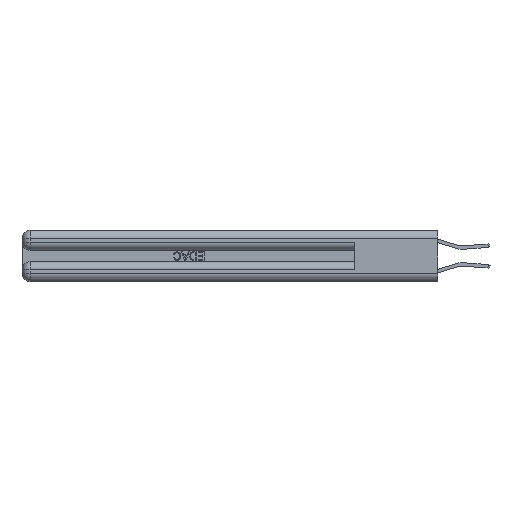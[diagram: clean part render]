
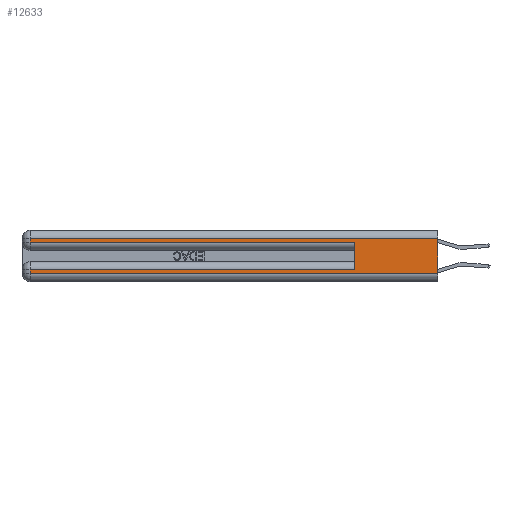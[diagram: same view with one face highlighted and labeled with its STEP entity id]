
A CAD part, left-side view. The second image highlights one B-rep face of the part: STEP entity #12633.
In plain terms, the highlighted planar face has unit normal (-1, 0, 0).
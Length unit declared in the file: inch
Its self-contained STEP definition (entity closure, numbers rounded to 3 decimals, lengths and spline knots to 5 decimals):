
#462 = FACE_OUTER_BOUND ( 'NONE', #24017, .T. ) ;
#1166 = LINE ( 'NONE', #32086, #22992 ) ;
#1452 = DIRECTION ( 'NONE',  ( 0., 1., 0. ) ) ;
#1502 = DIRECTION ( 'NONE',  ( 1., 0., 0. ) ) ;
#1860 = VERTEX_POINT ( 'NONE', #12380 ) ;
#1952 = EDGE_CURVE ( 'NONE', #29639, #1860, #1166, .T. ) ;
#2369 = VERTEX_POINT ( 'NONE', #33771 ) ;
#2550 = DIRECTION ( 'NONE',  ( 0., 0., 1. ) ) ;
#3182 = EDGE_CURVE ( 'NONE', #1860, #25771, #23637, .T. ) ;
#3885 = VECTOR ( 'NONE', #21975, 39.37008 ) ;
#4434 = DIRECTION ( 'NONE',  ( 0., 0., -1. ) ) ;
#5107 = LINE ( 'NONE', #13346, #8447 ) ;
#5162 = VECTOR ( 'NONE', #10854, 39.37008 ) ;
#5503 = ORIENTED_EDGE ( 'NONE', *, *, #1952, .T. ) ;
#5693 = LINE ( 'NONE', #18627, #14894 ) ;
#6251 = ORIENTED_EDGE ( 'NONE', *, *, #6834, .T. ) ;
#6834 = EDGE_CURVE ( 'NONE', #17349, #29639, #7426, .T. ) ;
#6919 = CARTESIAN_POINT ( 'NONE',  ( 0., 0., 0.37 ) ) ;
#7426 = LINE ( 'NONE', #16946, #18758 ) ;
#8447 = VECTOR ( 'NONE', #13696, 39.37008 ) ;
#8939 = VECTOR ( 'NONE', #26498, 39.37008 ) ;
#9323 = CARTESIAN_POINT ( 'NONE',  ( 0., 2.94, 0.285 ) ) ;
#9407 = LINE ( 'NONE', #28762, #27426 ) ;
#10305 = EDGE_CURVE ( 'NONE', #17349, #32527, #5693, .T. ) ;
#10809 = EDGE_CURVE ( 'NONE', #22746, #25771, #9407, .T. ) ;
#10854 = DIRECTION ( 'NONE',  ( 0., -1., 0. ) ) ;
#11839 = LINE ( 'NONE', #31795, #8939 ) ;
#12380 = CARTESIAN_POINT ( 'NONE',  ( 0., 2.94, 0.06 ) ) ;
#12633 = ADVANCED_FACE ( 'NONE', ( #462 ), #33997, .F. ) ;
#13096 = AXIS2_PLACEMENT_3D ( 'NONE', #6919, #1502, #28227 ) ;
#13346 = CARTESIAN_POINT ( 'NONE',  ( 0., 2.94, 0.37 ) ) ;
#13696 = DIRECTION ( 'NONE',  ( 0., 0., -1. ) ) ;
#14707 = VERTEX_POINT ( 'NONE', #9323 ) ;
#14743 = LINE ( 'NONE', #30144, #3885 ) ;
#14894 = VECTOR ( 'NONE', #2550, 39.37008 ) ;
#16594 = DIRECTION ( 'NONE',  ( 0., 0., -1. ) ) ;
#16946 = CARTESIAN_POINT ( 'NONE',  ( 0., 0., 0.085 ) ) ;
#17349 = VERTEX_POINT ( 'NONE', #24232 ) ;
#18627 = CARTESIAN_POINT ( 'NONE',  ( 0., 0.6, 0.145 ) ) ;
#18758 = VECTOR ( 'NONE', #1452, 39.37008 ) ;
#20392 = EDGE_CURVE ( 'NONE', #14707, #32527, #11839, .T. ) ;
#21689 = EDGE_CURVE ( 'NONE', #2369, #14707, #5107, .T. ) ;
#21975 = DIRECTION ( 'NONE',  ( 0., 1., 0. ) ) ;
#22746 = VERTEX_POINT ( 'NONE', #26091 ) ;
#22992 = VECTOR ( 'NONE', #16594, 39.37008 ) ;
#23354 = ORIENTED_EDGE ( 'NONE', *, *, #10809, .F. ) ;
#23637 = LINE ( 'NONE', #28922, #5162 ) ;
#24017 = EDGE_LOOP ( 'NONE', ( #23354, #29425, #30616, #27935, #29615, #6251, #5503, #32444 ) ) ;
#24232 = CARTESIAN_POINT ( 'NONE',  ( 0., 0.6, 0.085 ) ) ;
#25771 = VERTEX_POINT ( 'NONE', #28058 ) ;
#26091 = CARTESIAN_POINT ( 'NONE',  ( 0., 0., 0.31 ) ) ;
#26498 = DIRECTION ( 'NONE',  ( 0., -1., 0. ) ) ;
#27426 = VECTOR ( 'NONE', #4434, 39.37008 ) ;
#27607 = EDGE_CURVE ( 'NONE', #22746, #2369, #14743, .T. ) ;
#27935 = ORIENTED_EDGE ( 'NONE', *, *, #20392, .T. ) ;
#28058 = CARTESIAN_POINT ( 'NONE',  ( 0., 0., 0.06 ) ) ;
#28227 = DIRECTION ( 'NONE',  ( 0., 0., -1. ) ) ;
#28762 = CARTESIAN_POINT ( 'NONE',  ( 0., 0., 0.37 ) ) ;
#28922 = CARTESIAN_POINT ( 'NONE',  ( 0., 0., 0.06 ) ) ;
#29425 = ORIENTED_EDGE ( 'NONE', *, *, #27607, .T. ) ;
#29615 = ORIENTED_EDGE ( 'NONE', *, *, #10305, .F. ) ;
#29639 = VERTEX_POINT ( 'NONE', #30849 ) ;
#30144 = CARTESIAN_POINT ( 'NONE',  ( 0., 0., 0.31 ) ) ;
#30616 = ORIENTED_EDGE ( 'NONE', *, *, #21689, .T. ) ;
#30849 = CARTESIAN_POINT ( 'NONE',  ( 0., 2.94, 0.085 ) ) ;
#31795 = CARTESIAN_POINT ( 'NONE',  ( 0., 0., 0.285 ) ) ;
#31828 = CARTESIAN_POINT ( 'NONE',  ( 0., 0.6, 0.285 ) ) ;
#32086 = CARTESIAN_POINT ( 'NONE',  ( 0., 2.94, 0.37 ) ) ;
#32444 = ORIENTED_EDGE ( 'NONE', *, *, #3182, .T. ) ;
#32527 = VERTEX_POINT ( 'NONE', #31828 ) ;
#33771 = CARTESIAN_POINT ( 'NONE',  ( 0., 2.94, 0.31 ) ) ;
#33997 = PLANE ( 'NONE',  #13096 ) ;
